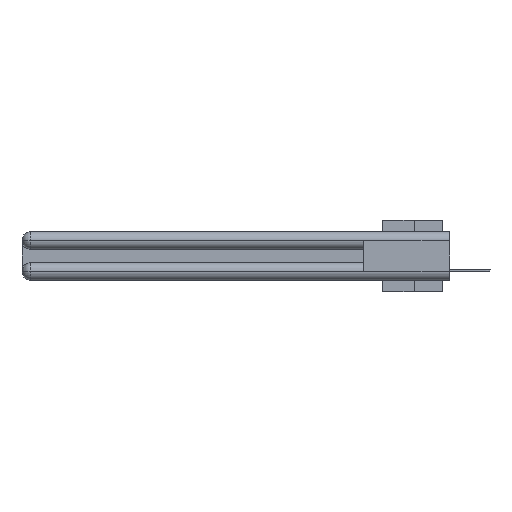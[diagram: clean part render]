
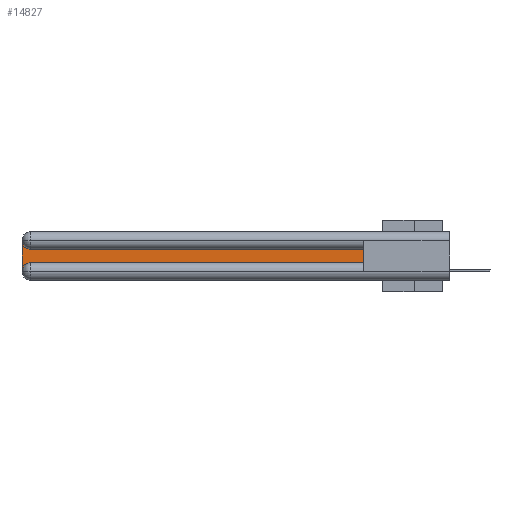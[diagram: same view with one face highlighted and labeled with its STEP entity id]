
A CAD part, left-side view. The second image highlights one B-rep face of the part: STEP entity #14827.
In plain terms, the highlighted planar face has unit normal (-1, 0, 0).
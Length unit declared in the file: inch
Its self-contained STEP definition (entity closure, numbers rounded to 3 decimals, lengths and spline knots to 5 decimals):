
#768 = CARTESIAN_POINT ( 'NONE',  ( 0.075, 0.6, -0.1225 ) ) ;
#1873 = CARTESIAN_POINT ( 'NONE',  ( 0.075, 2.94, -0.2175 ) ) ;
#2288 = ORIENTED_EDGE ( 'NONE', *, *, #15030, .T. ) ;
#2951 = CARTESIAN_POINT ( 'NONE',  ( 0.075, 2.94, -0.1225 ) ) ;
#3935 = ORIENTED_EDGE ( 'NONE', *, *, #12410, .T. ) ;
#4263 = VECTOR ( 'NONE', #32196, 39.37008 ) ;
#4551 = ORIENTED_EDGE ( 'NONE', *, *, #20361, .T. ) ;
#4954 = VECTOR ( 'NONE', #36989, 39.37008 ) ;
#5235 = LINE ( 'NONE', #26472, #4263 ) ;
#5260 = VERTEX_POINT ( 'NONE', #1873 ) ;
#6198 = FACE_OUTER_BOUND ( 'NONE', #17328, .T. ) ;
#6239 = ORIENTED_EDGE ( 'NONE', *, *, #28056, .T. ) ;
#6562 = CARTESIAN_POINT ( 'NONE',  ( 0.075, 3., -0.2175 ) ) ;
#6831 = ORIENTED_EDGE ( 'NONE', *, *, #36200, .T. ) ;
#6914 = DIRECTION ( 'NONE',  ( 0., 0., -1. ) ) ;
#8547 = AXIS2_PLACEMENT_3D ( 'NONE', #22301, #37670, #6914 ) ;
#8610 = DIRECTION ( 'NONE',  ( 1., 0., 0. ) ) ;
#11365 = VERTEX_POINT ( 'NONE', #21056 ) ;
#12378 = CIRCLE ( 'NONE', #8547, 0.06 ) ;
#12410 = EDGE_CURVE ( 'NONE', #25536, #11365, #35474, .T. ) ;
#12431 = DIRECTION ( 'NONE',  ( 0., 0., -1. ) ) ;
#12948 = LINE ( 'NONE', #28006, #29040 ) ;
#14827 = ADVANCED_FACE ( 'NONE', ( #6198 ), #20369, .F. ) ;
#15030 = EDGE_CURVE ( 'NONE', #30304, #25536, #21861, .T. ) ;
#17161 = CARTESIAN_POINT ( 'NONE',  ( 0.075, 3., -0.0625 ) ) ;
#17328 = EDGE_LOOP ( 'NONE', ( #4551, #2288, #3935, #6831, #36570, #6239 ) ) ;
#17671 = CARTESIAN_POINT ( 'NONE',  ( 0.075, 0.6, -0.1225 ) ) ;
#19102 = DIRECTION ( 'NONE',  ( 0., -1., 0. ) ) ;
#19284 = CARTESIAN_POINT ( 'NONE',  ( 0.075, 0.6, -0.2175 ) ) ;
#19354 = VERTEX_POINT ( 'NONE', #19284 ) ;
#20361 = EDGE_CURVE ( 'NONE', #35897, #30304, #37214, .T. ) ;
#20369 = PLANE ( 'NONE',  #35971 ) ;
#21056 = CARTESIAN_POINT ( 'NONE',  ( 0.075, 3., -0.2775 ) ) ;
#21861 = CIRCLE ( 'NONE', #27822, 0.06 ) ;
#22301 = CARTESIAN_POINT ( 'NONE',  ( 0.075, 2.94, -0.2775 ) ) ;
#22671 = VECTOR ( 'NONE', #12431, 39.37008 ) ;
#25536 = VERTEX_POINT ( 'NONE', #17161 ) ;
#26472 = CARTESIAN_POINT ( 'NONE',  ( 0.075, 0.6, -0.2175 ) ) ;
#26755 = CARTESIAN_POINT ( 'NONE',  ( 0.075, 2.94, -0.0625 ) ) ;
#26895 = DIRECTION ( 'NONE',  ( 0., 0., -1. ) ) ;
#27177 = EDGE_CURVE ( 'NONE', #5260, #19354, #12948, .T. ) ;
#27822 = AXIS2_PLACEMENT_3D ( 'NONE', #26755, #8610, #26895 ) ;
#28006 = CARTESIAN_POINT ( 'NONE',  ( 0.075, 0.6, -0.2175 ) ) ;
#28056 = EDGE_CURVE ( 'NONE', #19354, #35897, #5235, .T. ) ;
#29040 = VECTOR ( 'NONE', #19102, 39.37008 ) ;
#30304 = VERTEX_POINT ( 'NONE', #2951 ) ;
#32196 = DIRECTION ( 'NONE',  ( 0., 0., 1. ) ) ;
#32208 = DIRECTION ( 'NONE',  ( 1., 0., 0. ) ) ;
#32468 = DIRECTION ( 'NONE',  ( 0., 0., -1. ) ) ;
#32598 = CARTESIAN_POINT ( 'NONE',  ( 0.075, 3., -0.1225 ) ) ;
#35474 = LINE ( 'NONE', #6562, #22671 ) ;
#35897 = VERTEX_POINT ( 'NONE', #17671 ) ;
#35971 = AXIS2_PLACEMENT_3D ( 'NONE', #32598, #32208, #32468 ) ;
#36200 = EDGE_CURVE ( 'NONE', #11365, #5260, #12378, .T. ) ;
#36570 = ORIENTED_EDGE ( 'NONE', *, *, #27177, .T. ) ;
#36989 = DIRECTION ( 'NONE',  ( 0., 1., 0. ) ) ;
#37214 = LINE ( 'NONE', #768, #4954 ) ;
#37670 = DIRECTION ( 'NONE',  ( 1., 0., 0. ) ) ;
